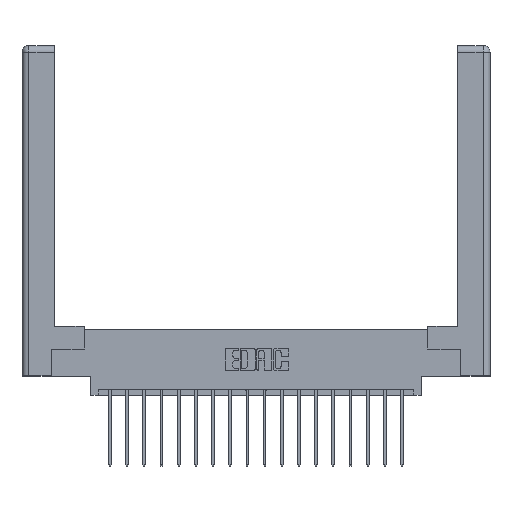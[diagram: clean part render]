
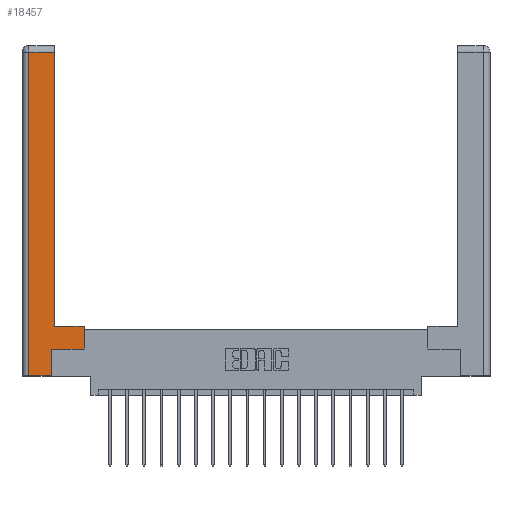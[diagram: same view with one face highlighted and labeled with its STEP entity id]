
A CAD part, top view. The second image highlights one B-rep face of the part: STEP entity #18457.
In plain terms, the highlighted planar face has unit normal (0, 0, 1).
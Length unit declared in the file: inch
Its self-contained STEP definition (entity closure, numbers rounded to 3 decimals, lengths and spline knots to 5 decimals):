
#393 = CARTESIAN_POINT ( 'NONE',  ( 0.565, 0.45, 0. ) ) ;
#452 = EDGE_CURVE ( 'NONE', #18184, #10418, #502, .T. ) ;
#502 = LINE ( 'NONE', #10330, #19475 ) ;
#629 = VECTOR ( 'NONE', #18940, 39.37008 ) ;
#1255 = VECTOR ( 'NONE', #18629, 39.37008 ) ;
#1523 = CARTESIAN_POINT ( 'NONE',  ( 0.565, 0.245, 0. ) ) ;
#1902 = VERTEX_POINT ( 'NONE', #18216 ) ;
#2193 = CARTESIAN_POINT ( 'NONE',  ( 0.265, 0.245, 0. ) ) ;
#2774 = VERTEX_POINT ( 'NONE', #2193 ) ;
#3480 = CARTESIAN_POINT ( 'NONE',  ( 0.295, 3., 0. ) ) ;
#3585 = CARTESIAN_POINT ( 'NONE',  ( 0.295, 2.94, 0. ) ) ;
#3811 = VERTEX_POINT ( 'NONE', #14160 ) ;
#3979 = DIRECTION ( 'NONE',  ( 0., 1., 0. ) ) ;
#4118 = CARTESIAN_POINT ( 'NONE',  ( 0.0615, 2.94, 0. ) ) ;
#4391 = VERTEX_POINT ( 'NONE', #4836 ) ;
#4836 = CARTESIAN_POINT ( 'NONE',  ( 0.565, 0.45, 0. ) ) ;
#5084 = EDGE_CURVE ( 'NONE', #10418, #1902, #13498, .T. ) ;
#5174 = DIRECTION ( 'NONE',  ( -1., 0., 0. ) ) ;
#5258 = ORIENTED_EDGE ( 'NONE', *, *, #452, .T. ) ;
#5270 = CARTESIAN_POINT ( 'NONE',  ( 0.565, 0.245, 0. ) ) ;
#5440 = EDGE_CURVE ( 'NONE', #1902, #3811, #8215, .T. ) ;
#5656 = DIRECTION ( 'NONE',  ( -1., 0., 0. ) ) ;
#5668 = DIRECTION ( 'NONE',  ( 1., 0., 0. ) ) ;
#6401 = LINE ( 'NONE', #5270, #629 ) ;
#6646 = CARTESIAN_POINT ( 'NONE',  ( 0.295, 0.45, 0. ) ) ;
#7147 = EDGE_CURVE ( 'NONE', #4391, #10574, #15379, .T. ) ;
#7154 = EDGE_CURVE ( 'NONE', #10574, #18184, #12715, .T. ) ;
#7505 = PLANE ( 'NONE',  #13079 ) ;
#8215 = LINE ( 'NONE', #16389, #14225 ) ;
#9053 = CARTESIAN_POINT ( 'NONE',  ( 0., 0., 0. ) ) ;
#9142 = VECTOR ( 'NONE', #14226, 39.37008 ) ;
#9915 = ORIENTED_EDGE ( 'NONE', *, *, #5440, .T. ) ;
#10330 = CARTESIAN_POINT ( 'NONE',  ( 0.0615, 2.94, 0. ) ) ;
#10418 = VERTEX_POINT ( 'NONE', #4118 ) ;
#10574 = VERTEX_POINT ( 'NONE', #15105 ) ;
#10581 = VECTOR ( 'NONE', #12590, 39.37008 ) ;
#10906 = EDGE_CURVE ( 'NONE', #15748, #4391, #13222, .T. ) ;
#11271 = VECTOR ( 'NONE', #5174, 39.37008 ) ;
#11551 = LINE ( 'NONE', #13145, #15650 ) ;
#11840 = ORIENTED_EDGE ( 'NONE', *, *, #5084, .T. ) ;
#12171 = DIRECTION ( 'NONE',  ( -1., 0., 0. ) ) ;
#12408 = ORIENTED_EDGE ( 'NONE', *, *, #7154, .T. ) ;
#12556 = CARTESIAN_POINT ( 'NONE',  ( 0.0615, 0., 0. ) ) ;
#12590 = DIRECTION ( 'NONE',  ( 0., 1., 0. ) ) ;
#12715 = LINE ( 'NONE', #3480, #9142 ) ;
#12893 = ORIENTED_EDGE ( 'NONE', *, *, #16950, .T. ) ;
#13079 = AXIS2_PLACEMENT_3D ( 'NONE', #9053, #15090, #12171 ) ;
#13145 = CARTESIAN_POINT ( 'NONE',  ( 0.265, 0.245, 0. ) ) ;
#13215 = FACE_OUTER_BOUND ( 'NONE', #13216, .T. ) ;
#13216 = EDGE_LOOP ( 'NONE', ( #12408, #5258, #11840, #9915, #12893, #15855, #13487, #13366 ) ) ;
#13222 = LINE ( 'NONE', #393, #10581 ) ;
#13366 = ORIENTED_EDGE ( 'NONE', *, *, #7147, .T. ) ;
#13487 = ORIENTED_EDGE ( 'NONE', *, *, #10906, .T. ) ;
#13498 = LINE ( 'NONE', #12556, #1255 ) ;
#14160 = CARTESIAN_POINT ( 'NONE',  ( 0.265, 0., 0. ) ) ;
#14225 = VECTOR ( 'NONE', #5668, 39.37008 ) ;
#14226 = DIRECTION ( 'NONE',  ( 0., 1., 0. ) ) ;
#14649 = EDGE_CURVE ( 'NONE', #2774, #15748, #6401, .T. ) ;
#15090 = DIRECTION ( 'NONE',  ( 0., 0., -1. ) ) ;
#15105 = CARTESIAN_POINT ( 'NONE',  ( 0.295, 0.45, 0. ) ) ;
#15379 = LINE ( 'NONE', #6646, #11271 ) ;
#15650 = VECTOR ( 'NONE', #3979, 39.37008 ) ;
#15748 = VERTEX_POINT ( 'NONE', #1523 ) ;
#15855 = ORIENTED_EDGE ( 'NONE', *, *, #14649, .T. ) ;
#16389 = CARTESIAN_POINT ( 'NONE',  ( 0.265, 0., 0. ) ) ;
#16950 = EDGE_CURVE ( 'NONE', #3811, #2774, #11551, .T. ) ;
#18184 = VERTEX_POINT ( 'NONE', #3585 ) ;
#18216 = CARTESIAN_POINT ( 'NONE',  ( 0.0615, 0., 0. ) ) ;
#18457 = ADVANCED_FACE ( 'NONE', ( #13215 ), #7505, .F. ) ;
#18629 = DIRECTION ( 'NONE',  ( 0., -1., 0. ) ) ;
#18940 = DIRECTION ( 'NONE',  ( 1., 0., 0. ) ) ;
#19475 = VECTOR ( 'NONE', #5656, 39.37008 ) ;
